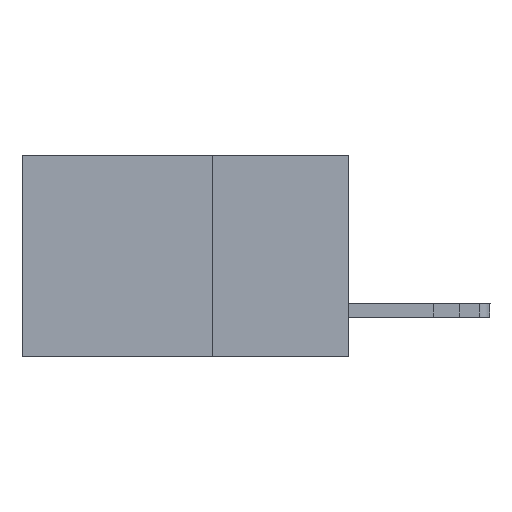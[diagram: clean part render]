
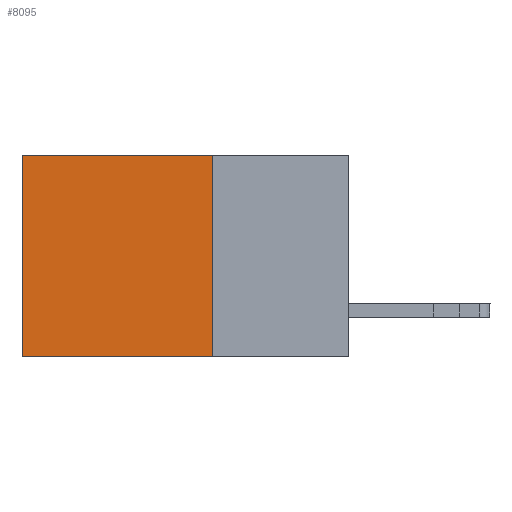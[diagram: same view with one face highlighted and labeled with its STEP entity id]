
A CAD part, left-side view. The second image highlights one B-rep face of the part: STEP entity #8095.
In plain terms, the highlighted planar face has unit normal (-1, 0, 0).
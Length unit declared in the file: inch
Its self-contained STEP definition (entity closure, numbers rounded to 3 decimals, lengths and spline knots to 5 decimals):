
#163 = ORIENTED_EDGE ( 'NONE', *, *, #3034, .T. ) ;
#212 = FACE_OUTER_BOUND ( 'NONE', #3570, .T. ) ;
#260 = DIRECTION ( 'NONE',  ( 0., 0., -1. ) ) ;
#276 = CARTESIAN_POINT ( 'NONE',  ( 0.2615, 0.6, -0.37 ) ) ;
#654 = CARTESIAN_POINT ( 'NONE',  ( 0.2615, 0.25, -0.37 ) ) ;
#827 = AXIS2_PLACEMENT_3D ( 'NONE', #4087, #7153, #260 ) ;
#979 = VECTOR ( 'NONE', #2206, 39.37008 ) ;
#1283 = CARTESIAN_POINT ( 'NONE',  ( 0.2615, 0.6, 0. ) ) ;
#2206 = DIRECTION ( 'NONE',  ( 0., 1., 0. ) ) ;
#2776 = LINE ( 'NONE', #5771, #5229 ) ;
#3034 = EDGE_CURVE ( 'NONE', #6267, #7892, #3736, .T. ) ;
#3464 = EDGE_CURVE ( 'NONE', #4341, #6267, #8942, .T. ) ;
#3570 = EDGE_LOOP ( 'NONE', ( #163, #8948, #7980, #6742 ) ) ;
#3736 = LINE ( 'NONE', #6739, #4541 ) ;
#3876 = CARTESIAN_POINT ( 'NONE',  ( 0.2615, 0.25, 0. ) ) ;
#4055 = DIRECTION ( 'NONE',  ( 0., 0., -1. ) ) ;
#4087 = CARTESIAN_POINT ( 'NONE',  ( 0.2615, 0.25, -0.37 ) ) ;
#4341 = VERTEX_POINT ( 'NONE', #3876 ) ;
#4541 = VECTOR ( 'NONE', #4055, 39.37008 ) ;
#4771 = LINE ( 'NONE', #6304, #7697 ) ;
#5229 = VECTOR ( 'NONE', #5877, 39.37008 ) ;
#5258 = CARTESIAN_POINT ( 'NONE',  ( 0.2615, 0.25, 0. ) ) ;
#5755 = EDGE_CURVE ( 'NONE', #4341, #8250, #4771, .T. ) ;
#5771 = CARTESIAN_POINT ( 'NONE',  ( 0.2615, 0.25, -0.37 ) ) ;
#5877 = DIRECTION ( 'NONE',  ( 0., 1., 0. ) ) ;
#6267 = VERTEX_POINT ( 'NONE', #1283 ) ;
#6304 = CARTESIAN_POINT ( 'NONE',  ( 0.2615, 0.25, -0.37 ) ) ;
#6739 = CARTESIAN_POINT ( 'NONE',  ( 0.2615, 0.6, -0.37 ) ) ;
#6742 = ORIENTED_EDGE ( 'NONE', *, *, #3464, .T. ) ;
#7153 = DIRECTION ( 'NONE',  ( 1., 0., 0. ) ) ;
#7201 = EDGE_CURVE ( 'NONE', #8250, #7892, #2776, .T. ) ;
#7697 = VECTOR ( 'NONE', #7726, 39.37008 ) ;
#7726 = DIRECTION ( 'NONE',  ( 0., 0., -1. ) ) ;
#7787 = PLANE ( 'NONE',  #827 ) ;
#7892 = VERTEX_POINT ( 'NONE', #276 ) ;
#7980 = ORIENTED_EDGE ( 'NONE', *, *, #5755, .F. ) ;
#8095 = ADVANCED_FACE ( 'NONE', ( #212 ), #7787, .F. ) ;
#8250 = VERTEX_POINT ( 'NONE', #654 ) ;
#8942 = LINE ( 'NONE', #5258, #979 ) ;
#8948 = ORIENTED_EDGE ( 'NONE', *, *, #7201, .F. ) ;
